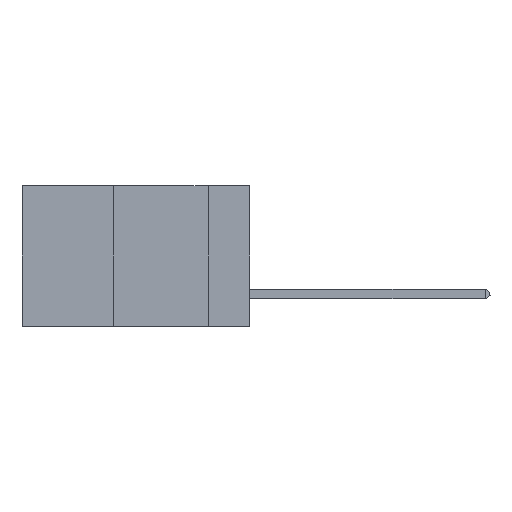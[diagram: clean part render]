
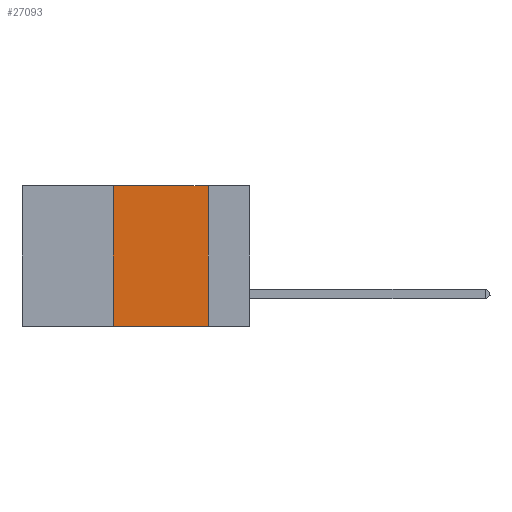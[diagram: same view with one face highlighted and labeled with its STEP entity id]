
A CAD part, left-side view. The second image highlights one B-rep face of the part: STEP entity #27093.
In plain terms, the highlighted planar face has unit normal (-1, 0, 0).
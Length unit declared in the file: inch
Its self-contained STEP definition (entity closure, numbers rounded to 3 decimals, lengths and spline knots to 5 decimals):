
#28 = FACE_OUTER_BOUND ( 'NONE', #39435, .T. ) ;
#1575 = ORIENTED_EDGE ( 'NONE', *, *, #10902, .F. ) ;
#1588 = CARTESIAN_POINT ( 'NONE',  ( 0., 0.6, 0. ) ) ;
#3020 = LINE ( 'NONE', #1588, #42730 ) ;
#3541 = ORIENTED_EDGE ( 'NONE', *, *, #12833, .F. ) ;
#6895 = LINE ( 'NONE', #13519, #45449 ) ;
#8050 = DIRECTION ( 'NONE',  ( 0., 0., -1. ) ) ;
#10902 = EDGE_CURVE ( 'NONE', #38575, #35961, #3020, .T. ) ;
#11763 = VERTEX_POINT ( 'NONE', #14822 ) ;
#12321 = EDGE_CURVE ( 'NONE', #19383, #11763, #12747, .T. ) ;
#12747 = LINE ( 'NONE', #29203, #42545 ) ;
#12833 = EDGE_CURVE ( 'NONE', #19383, #38575, #6895, .T. ) ;
#13519 = CARTESIAN_POINT ( 'NONE',  ( 0., 0.36, 0. ) ) ;
#14822 = CARTESIAN_POINT ( 'NONE',  ( 0., 0.11, -0.37 ) ) ;
#16038 = PLANE ( 'NONE',  #33457 ) ;
#19383 = VERTEX_POINT ( 'NONE', #42185 ) ;
#19672 = DIRECTION ( 'NONE',  ( 0., -1., 0. ) ) ;
#23026 = CARTESIAN_POINT ( 'NONE',  ( 0., 0.6, 0. ) ) ;
#24534 = LINE ( 'NONE', #36082, #36218 ) ;
#25010 = DIRECTION ( 'NONE',  ( 0., 0., -1. ) ) ;
#25131 = DIRECTION ( 'NONE',  ( 0., -1., 0. ) ) ;
#26457 = DIRECTION ( 'NONE',  ( 1., 0., 0. ) ) ;
#26735 = EDGE_CURVE ( 'NONE', #35961, #11763, #24534, .T. ) ;
#27093 = ADVANCED_FACE ( 'NONE', ( #28 ), #16038, .F. ) ;
#28634 = ORIENTED_EDGE ( 'NONE', *, *, #26735, .F. ) ;
#29203 = CARTESIAN_POINT ( 'NONE',  ( 0., 0.6, -0.37 ) ) ;
#33155 = ORIENTED_EDGE ( 'NONE', *, *, #12321, .T. ) ;
#33457 = AXIS2_PLACEMENT_3D ( 'NONE', #23026, #26457, #8050 ) ;
#35961 = VERTEX_POINT ( 'NONE', #47811 ) ;
#36082 = CARTESIAN_POINT ( 'NONE',  ( 0., 0.11, 0. ) ) ;
#36218 = VECTOR ( 'NONE', #25010, 39.37008 ) ;
#38575 = VERTEX_POINT ( 'NONE', #39163 ) ;
#39163 = CARTESIAN_POINT ( 'NONE',  ( 0., 0.36, 0. ) ) ;
#39435 = EDGE_LOOP ( 'NONE', ( #28634, #1575, #3541, #33155 ) ) ;
#39939 = DIRECTION ( 'NONE',  ( 0., 0., 1. ) ) ;
#42185 = CARTESIAN_POINT ( 'NONE',  ( 0., 0.36, -0.37 ) ) ;
#42545 = VECTOR ( 'NONE', #25131, 39.37008 ) ;
#42730 = VECTOR ( 'NONE', #19672, 39.37008 ) ;
#45449 = VECTOR ( 'NONE', #39939, 39.37008 ) ;
#47811 = CARTESIAN_POINT ( 'NONE',  ( 0., 0.11, 0. ) ) ;
